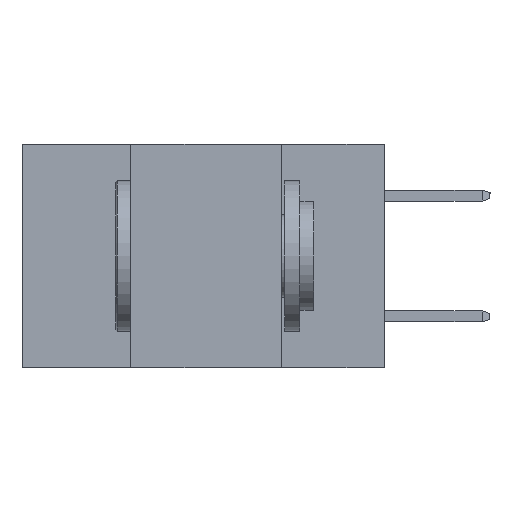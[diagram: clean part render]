
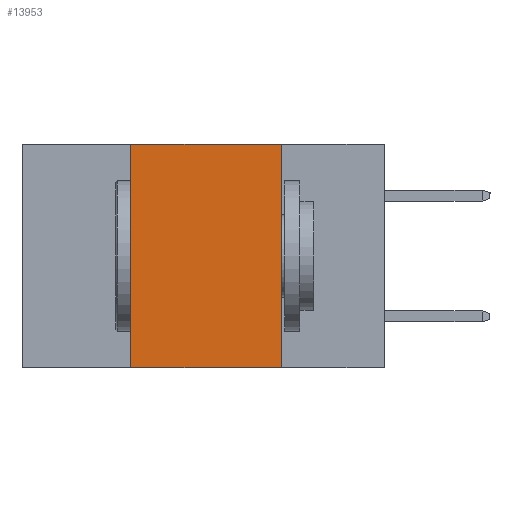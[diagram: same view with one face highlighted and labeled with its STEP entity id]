
A CAD part, left-side view. The second image highlights one B-rep face of the part: STEP entity #13953.
In plain terms, the highlighted planar face has unit normal (-1, 0, 0).
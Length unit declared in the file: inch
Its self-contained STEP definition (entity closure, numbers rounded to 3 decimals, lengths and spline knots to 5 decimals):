
#162 = DIRECTION ( 'NONE',  ( 0., 0., -1. ) ) ;
#292 = DIRECTION ( 'NONE',  ( 0., 0., 1. ) ) ;
#760 = EDGE_CURVE ( 'NONE', #4861, #3108, #2680, .T. ) ;
#1825 = CARTESIAN_POINT ( 'NONE',  ( 0., 0.42, 0. ) ) ;
#2094 = PLANE ( 'NONE',  #15875 ) ;
#2680 = LINE ( 'NONE', #17915, #11236 ) ;
#3108 = VERTEX_POINT ( 'NONE', #19332 ) ;
#3883 = CARTESIAN_POINT ( 'NONE',  ( 0., 0.42, -0.37 ) ) ;
#4595 = VERTEX_POINT ( 'NONE', #6738 ) ;
#4766 = CARTESIAN_POINT ( 'NONE',  ( 0., 0.42, -0.37 ) ) ;
#4861 = VERTEX_POINT ( 'NONE', #4766 ) ;
#5163 = ORIENTED_EDGE ( 'NONE', *, *, #13914, .F. ) ;
#6096 = EDGE_CURVE ( 'NONE', #20160, #4595, #11484, .T. ) ;
#6316 = DIRECTION ( 'NONE',  ( 0., -1., 0. ) ) ;
#6689 = CARTESIAN_POINT ( 'NONE',  ( 0., 0.17, -0.37 ) ) ;
#6738 = CARTESIAN_POINT ( 'NONE',  ( 0., 0.17, 0. ) ) ;
#7165 = FACE_OUTER_BOUND ( 'NONE', #20079, .T. ) ;
#7205 = ORIENTED_EDGE ( 'NONE', *, *, #6096, .F. ) ;
#7281 = DIRECTION ( 'NONE',  ( 1., 0., 0. ) ) ;
#11236 = VECTOR ( 'NONE', #21499, 39.37008 ) ;
#11484 = LINE ( 'NONE', #16914, #18460 ) ;
#11901 = VECTOR ( 'NONE', #292, 39.37008 ) ;
#12353 = CARTESIAN_POINT ( 'NONE',  ( 0., 0.6, 0. ) ) ;
#13914 = EDGE_CURVE ( 'NONE', #4861, #20160, #20714, .T. ) ;
#13953 = ADVANCED_FACE ( 'NONE', ( #7165 ), #2094, .F. ) ;
#15706 = LINE ( 'NONE', #6689, #20595 ) ;
#15875 = AXIS2_PLACEMENT_3D ( 'NONE', #12353, #7281, #19242 ) ;
#16328 = EDGE_CURVE ( 'NONE', #4595, #3108, #15706, .T. ) ;
#16914 = CARTESIAN_POINT ( 'NONE',  ( 0., 0.6, 0. ) ) ;
#17915 = CARTESIAN_POINT ( 'NONE',  ( 0., 0.6, -0.37 ) ) ;
#18072 = ORIENTED_EDGE ( 'NONE', *, *, #16328, .F. ) ;
#18460 = VECTOR ( 'NONE', #6316, 39.37008 ) ;
#19242 = DIRECTION ( 'NONE',  ( 0., 0., -1. ) ) ;
#19332 = CARTESIAN_POINT ( 'NONE',  ( 0., 0.17, -0.37 ) ) ;
#20079 = EDGE_LOOP ( 'NONE', ( #18072, #7205, #5163, #22245 ) ) ;
#20160 = VERTEX_POINT ( 'NONE', #1825 ) ;
#20595 = VECTOR ( 'NONE', #162, 39.37008 ) ;
#20714 = LINE ( 'NONE', #3883, #11901 ) ;
#21499 = DIRECTION ( 'NONE',  ( 0., -1., 0. ) ) ;
#22245 = ORIENTED_EDGE ( 'NONE', *, *, #760, .T. ) ;
